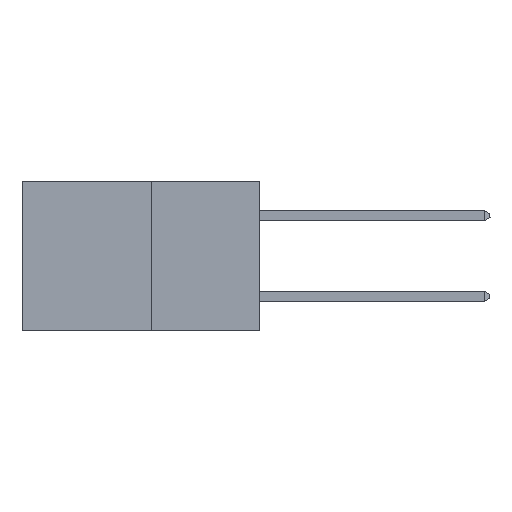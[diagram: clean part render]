
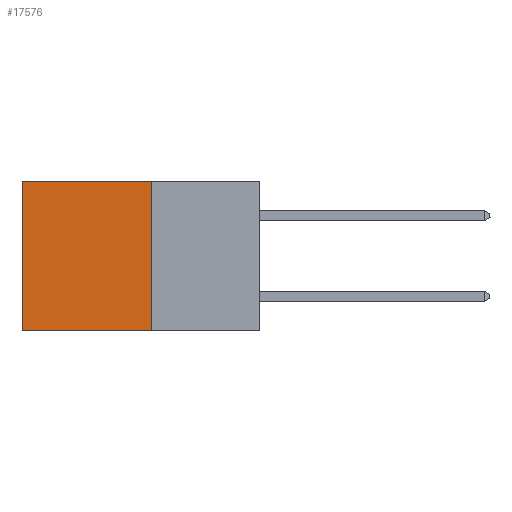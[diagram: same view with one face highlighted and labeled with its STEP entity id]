
A CAD part, left-side view. The second image highlights one B-rep face of the part: STEP entity #17576.
In plain terms, the highlighted planar face has unit normal (-1, 0, 0).
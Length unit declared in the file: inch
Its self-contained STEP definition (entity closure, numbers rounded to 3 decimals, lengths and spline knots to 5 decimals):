
#614 = EDGE_LOOP ( 'NONE', ( #2584, #13110, #13305, #12141 ) ) ;
#1167 = DIRECTION ( 'NONE',  ( 1., 0., 0. ) ) ;
#2038 = EDGE_CURVE ( 'NONE', #16524, #14799, #13840, .T. ) ;
#2584 = ORIENTED_EDGE ( 'NONE', *, *, #14255, .T. ) ;
#2719 = AXIS2_PLACEMENT_3D ( 'NONE', #9836, #1167, #11279 ) ;
#2780 = VECTOR ( 'NONE', #6127, 39.37008 ) ;
#3229 = LINE ( 'NONE', #16145, #2780 ) ;
#3582 = CARTESIAN_POINT ( 'NONE',  ( 0.277, 0.27, 0. ) ) ;
#3774 = VECTOR ( 'NONE', #4785, 39.37008 ) ;
#4425 = EDGE_CURVE ( 'NONE', #10175, #8624, #15386, .T. ) ;
#4489 = VECTOR ( 'NONE', #10519, 39.37008 ) ;
#4590 = CARTESIAN_POINT ( 'NONE',  ( 0.277, 0.59, -0.37 ) ) ;
#4785 = DIRECTION ( 'NONE',  ( 0., 1., 0. ) ) ;
#6119 = VECTOR ( 'NONE', #8749, 39.37008 ) ;
#6127 = DIRECTION ( 'NONE',  ( 0., 0., -1. ) ) ;
#6938 = PLANE ( 'NONE',  #2719 ) ;
#7634 = CARTESIAN_POINT ( 'NONE',  ( 0.277, 0.59, -0.37 ) ) ;
#7869 = CARTESIAN_POINT ( 'NONE',  ( 0.277, 0.27, 0. ) ) ;
#8344 = LINE ( 'NONE', #7634, #4489 ) ;
#8624 = VERTEX_POINT ( 'NONE', #12897 ) ;
#8749 = DIRECTION ( 'NONE',  ( 0., 1., 0. ) ) ;
#9210 = EDGE_CURVE ( 'NONE', #10175, #16524, #3229, .T. ) ;
#9836 = CARTESIAN_POINT ( 'NONE',  ( 0.277, 0.27, -0.37 ) ) ;
#9925 = FACE_OUTER_BOUND ( 'NONE', #614, .T. ) ;
#10175 = VERTEX_POINT ( 'NONE', #7869 ) ;
#10519 = DIRECTION ( 'NONE',  ( 0., 0., -1. ) ) ;
#11279 = DIRECTION ( 'NONE',  ( 0., 0., -1. ) ) ;
#12141 = ORIENTED_EDGE ( 'NONE', *, *, #4425, .T. ) ;
#12897 = CARTESIAN_POINT ( 'NONE',  ( 0.277, 0.59, 0. ) ) ;
#13110 = ORIENTED_EDGE ( 'NONE', *, *, #2038, .F. ) ;
#13305 = ORIENTED_EDGE ( 'NONE', *, *, #9210, .F. ) ;
#13840 = LINE ( 'NONE', #15264, #6119 ) ;
#14255 = EDGE_CURVE ( 'NONE', #8624, #14799, #8344, .T. ) ;
#14799 = VERTEX_POINT ( 'NONE', #4590 ) ;
#14864 = CARTESIAN_POINT ( 'NONE',  ( 0.277, 0.27, -0.37 ) ) ;
#15264 = CARTESIAN_POINT ( 'NONE',  ( 0.277, 0.27, -0.37 ) ) ;
#15386 = LINE ( 'NONE', #3582, #3774 ) ;
#16145 = CARTESIAN_POINT ( 'NONE',  ( 0.277, 0.27, -0.37 ) ) ;
#16524 = VERTEX_POINT ( 'NONE', #14864 ) ;
#17576 = ADVANCED_FACE ( 'NONE', ( #9925 ), #6938, .F. ) ;
